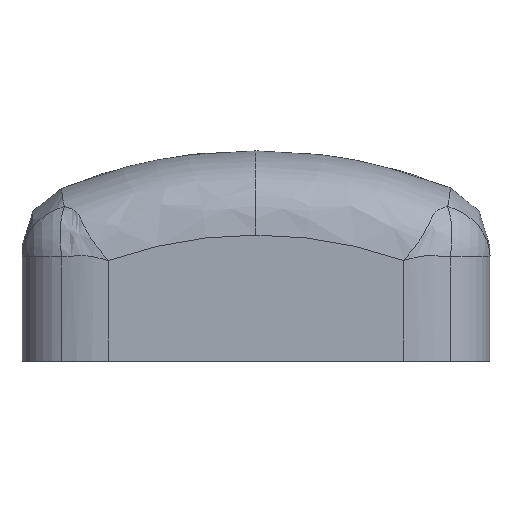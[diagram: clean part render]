
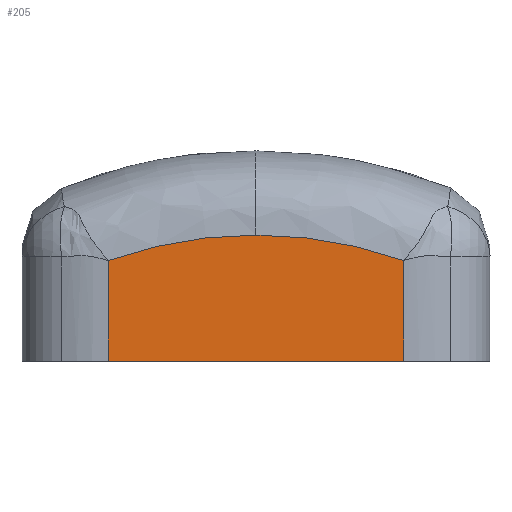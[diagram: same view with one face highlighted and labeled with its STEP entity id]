
A CAD part, left-side view. The second image highlights one B-rep face of the part: STEP entity #205.
In plain terms, the highlighted planar face has unit normal (-1, 0, 0).
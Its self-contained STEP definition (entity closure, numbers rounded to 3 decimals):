
#188 = CARTESIAN_POINT ( 'NONE',  ( -84.042, 11.717, 0. ) ) ;
#200 = CARTESIAN_POINT ( 'NONE',  ( -84.042, -11.717, 7.98 ) ) ;
#201 = CARTESIAN_POINT ( 'NONE',  ( -84.042, -11.717, 0. ) ) ;
#205 = ADVANCED_FACE ( 'NONE', ( #1012 ), #1885, .F. ) ;
#292 = AXIS2_PLACEMENT_3D ( 'NONE', #1425, #1420, #1418 ) ;
#474 = EDGE_LOOP ( 'NONE', ( #1586, #1762, #1040, #1349, #1290 ) ) ;
#530 = AXIS2_PLACEMENT_3D ( 'NONE', #1736, #1713, #1687 ) ;
#795 = VECTOR ( 'NONE', #1973, 1000. ) ;
#912 = LINE ( 'NONE', #1983, #795 ) ;
#1012 = FACE_OUTER_BOUND ( 'NONE', #474, .T. ) ;
#1040 = ORIENTED_EDGE ( 'NONE', *, *, #1774, .T. ) ;
#1091 = VERTEX_POINT ( 'NONE', #201 ) ;
#1140 = VERTEX_POINT ( 'NONE', #200 ) ;
#1161 = LINE ( 'NONE', #1335, #1169 ) ;
#1169 = VECTOR ( 'NONE', #1404, 1000. ) ;
#1279 = CARTESIAN_POINT ( 'NONE',  ( -84.042, 11.717, 7.98 ) ) ;
#1290 = ORIENTED_EDGE ( 'NONE', *, *, #1839, .T. ) ;
#1306 = VECTOR ( 'NONE', #1622, 1000. ) ;
#1335 = CARTESIAN_POINT ( 'NONE',  ( -84.042, 11.717, 0. ) ) ;
#1349 = ORIENTED_EDGE ( 'NONE', *, *, #1870, .T. ) ;
#1394 = CIRCLE ( 'NONE', #292, 35. ) ;
#1404 = DIRECTION ( 'NONE',  ( 0., -1., 0. ) ) ;
#1407 = LINE ( 'NONE', #1639, #1306 ) ;
#1418 = DIRECTION ( 'NONE',  ( 0., 1., 0. ) ) ;
#1420 = DIRECTION ( 'NONE',  ( -1., 0., 0. ) ) ;
#1425 = CARTESIAN_POINT ( 'NONE',  ( -84.042, 0., -25. ) ) ;
#1445 = CIRCLE ( 'NONE', #530, 35. ) ;
#1476 = VERTEX_POINT ( 'NONE', #1995 ) ;
#1515 = EDGE_CURVE ( 'NONE', #1140, #1091, #912, .T. ) ;
#1586 = ORIENTED_EDGE ( 'NONE', *, *, #1879, .T. ) ;
#1622 = DIRECTION ( 'NONE',  ( 0., 0., -1. ) ) ;
#1639 = CARTESIAN_POINT ( 'NONE',  ( -84.042, 11.717, 5. ) ) ;
#1682 = VERTEX_POINT ( 'NONE', #1279 ) ;
#1687 = DIRECTION ( 'NONE',  ( 0., 1., 0. ) ) ;
#1713 = DIRECTION ( 'NONE',  ( -1., 0., 0. ) ) ;
#1736 = CARTESIAN_POINT ( 'NONE',  ( -84.042, 0., -25. ) ) ;
#1762 = ORIENTED_EDGE ( 'NONE', *, *, #1515, .F. ) ;
#1768 = VERTEX_POINT ( 'NONE', #188 ) ;
#1774 = EDGE_CURVE ( 'NONE', #1140, #1476, #1445, .T. ) ;
#1798 = CARTESIAN_POINT ( 'NONE',  ( -84.042, 11.717, 5. ) ) ;
#1839 = EDGE_CURVE ( 'NONE', #1682, #1768, #1407, .T. ) ;
#1850 = DIRECTION ( 'NONE',  ( 0., 1., 0. ) ) ;
#1860 = DIRECTION ( 'NONE',  ( 1., 0., 0. ) ) ;
#1870 = EDGE_CURVE ( 'NONE', #1476, #1682, #1394, .T. ) ;
#1879 = EDGE_CURVE ( 'NONE', #1768, #1091, #1161, .T. ) ;
#1885 = PLANE ( 'NONE',  #1974 ) ;
#1973 = DIRECTION ( 'NONE',  ( 0., 0., -1. ) ) ;
#1974 = AXIS2_PLACEMENT_3D ( 'NONE', #1798, #1860, #1850 ) ;
#1983 = CARTESIAN_POINT ( 'NONE',  ( -84.042, -11.717, 5. ) ) ;
#1995 = CARTESIAN_POINT ( 'NONE',  ( -84.042, 0.001, 10. ) ) ;
